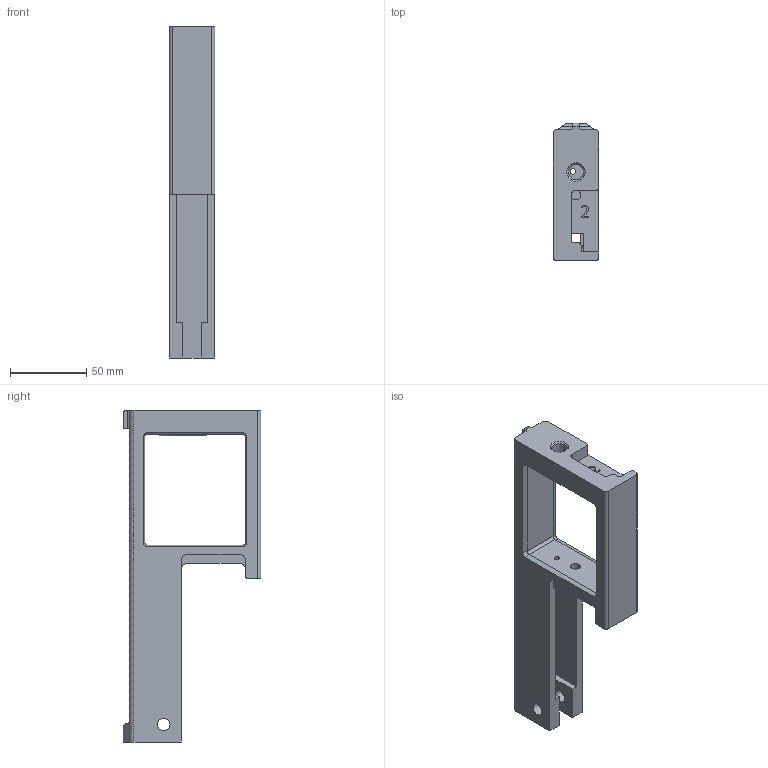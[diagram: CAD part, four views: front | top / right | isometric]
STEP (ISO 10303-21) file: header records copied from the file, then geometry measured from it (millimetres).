
FILE_DESCRIPTION((''),'2;1');
FILE_NAME('PM522Frame2.stp','2015-10-01T18:15:51',('JamesRPatrick'),(''),'Autodesk Inventor 2012','Autodesk Inventor 2012','');
FILE_SCHEMA(('AUTOMOTIVE_DESIGN { 1 0 10303 214 1 1 1 1 }'));
Length unit declared in the file: millimetre
Products named in the file (1): PM522Frame2
Bounding box: 30 x 90 x 217.5 mm (x, y, z)
Volume: 171557.2 mm3; surface area: 51830.7 mm2
Topology: 1 solids, 1 shells, 382 faces, 1053 edges, 695 vertices
Faces by surface type: plane 247, bspline 79, cylinder 44, cone 12
Full cylindrical faces by diameter (mm): 3.5 x1, 6.4 x2, 8.2 x2, 10 x1, 14 x1
Entity records: 13013 total; most frequent: CARTESIAN_POINT 3389, ORIENTED_EDGE 2086, DIRECTION 1595, EDGE_CURVE 1043, VECTOR 781, LINE 781, VERTEX_POINT 694, EDGE_LOOP 429
